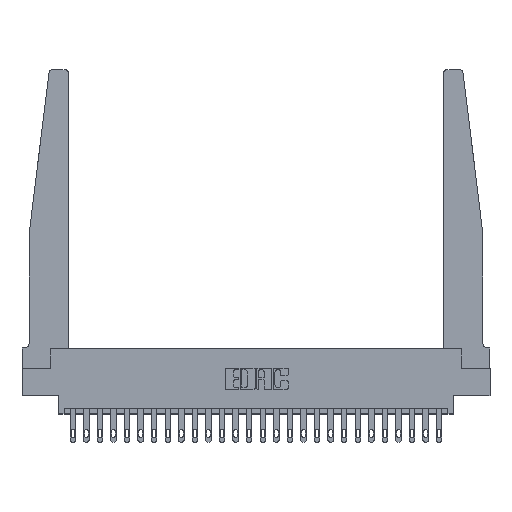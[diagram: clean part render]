
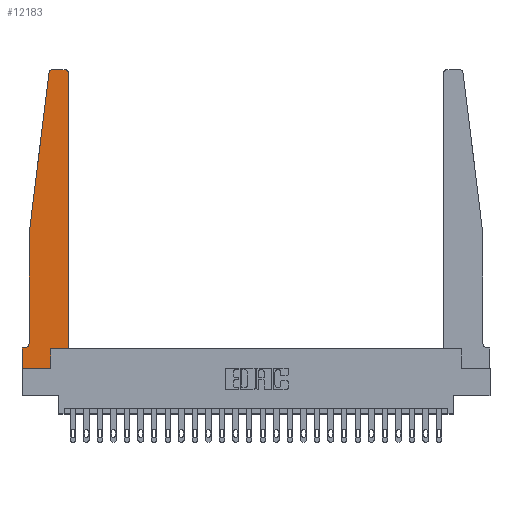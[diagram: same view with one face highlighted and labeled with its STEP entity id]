
A CAD part, top view. The second image highlights one B-rep face of the part: STEP entity #12183.
In plain terms, the highlighted planar face has unit normal (0, 0, 1).
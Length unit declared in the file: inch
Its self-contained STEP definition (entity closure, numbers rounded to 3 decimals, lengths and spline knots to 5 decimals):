
#21 = VECTOR ( 'NONE', #12403, 39.37008 ) ;
#316 = DIRECTION ( 'NONE',  ( 0., -1., 0. ) ) ;
#519 = VERTEX_POINT ( 'NONE', #16243 ) ;
#583 = VECTOR ( 'NONE', #2720, 39.37008 ) ;
#841 = ORIENTED_EDGE ( 'NONE', *, *, #5071, .T. ) ;
#879 = LINE ( 'NONE', #22635, #21383 ) ;
#904 = CARTESIAN_POINT ( 'NONE',  ( 0.2605, 0.18, 0.37 ) ) ;
#988 = CARTESIAN_POINT ( 'NONE',  ( 0.065, 1.25, 0.37 ) ) ;
#1230 = CARTESIAN_POINT ( 'NONE',  ( 0.425, 0.18, 0.37 ) ) ;
#1241 = ORIENTED_EDGE ( 'NONE', *, *, #4500, .T. ) ;
#1388 = CIRCLE ( 'NONE', #5923, 0.05 ) ;
#1727 = CARTESIAN_POINT ( 'NONE',  ( 0.27653, 2.72, 0.37 ) ) ;
#1816 = LINE ( 'NONE', #7747, #4727 ) ;
#1853 = EDGE_CURVE ( 'NONE', #3361, #12237, #2356, .T. ) ;
#2356 = LINE ( 'NONE', #21667, #24322 ) ;
#2442 = CARTESIAN_POINT ( 'NONE',  ( 0.065, 1.25, 0.37 ) ) ;
#2459 = LINE ( 'NONE', #904, #8389 ) ;
#2460 = FACE_OUTER_BOUND ( 'NONE', #20268, .T. ) ;
#2645 = AXIS2_PLACEMENT_3D ( 'NONE', #1727, #7530, #21415 ) ;
#2720 = DIRECTION ( 'NONE',  ( 0., 1., 0. ) ) ;
#3138 = VERTEX_POINT ( 'NONE', #988 ) ;
#3288 = ORIENTED_EDGE ( 'NONE', *, *, #16578, .T. ) ;
#3361 = VERTEX_POINT ( 'NONE', #10367 ) ;
#3386 = DIRECTION ( 'NONE',  ( 0., 0., 1. ) ) ;
#3584 = EDGE_CURVE ( 'NONE', #12237, #519, #18254, .T. ) ;
#3798 = CARTESIAN_POINT ( 'NONE',  ( 0.065, 0.1875, 0.37 ) ) ;
#3959 = VECTOR ( 'NONE', #316, 39.37008 ) ;
#4500 = EDGE_CURVE ( 'NONE', #24695, #19992, #1388, .T. ) ;
#4727 = VECTOR ( 'NONE', #9683, 39.37008 ) ;
#4728 = LINE ( 'NONE', #1230, #13817 ) ;
#5071 = EDGE_CURVE ( 'NONE', #15024, #10691, #21679, .T. ) ;
#5421 = CARTESIAN_POINT ( 'NONE',  ( 0.2605, 0., 0.37 ) ) ;
#5449 = EDGE_CURVE ( 'NONE', #9750, #23066, #2459, .T. ) ;
#5635 = DIRECTION ( 'NONE',  ( 0., 0., -1. ) ) ;
#5793 = CIRCLE ( 'NONE', #16869, 0.03 ) ;
#5923 = AXIS2_PLACEMENT_3D ( 'NONE', #23272, #5635, #13356 ) ;
#6958 = DIRECTION ( 'NONE',  ( 0., 1., 0. ) ) ;
#7075 = ORIENTED_EDGE ( 'NONE', *, *, #1853, .T. ) ;
#7202 = EDGE_CURVE ( 'NONE', #10691, #9750, #879, .T. ) ;
#7530 = DIRECTION ( 'NONE',  ( 0., 0., 1. ) ) ;
#7678 = LINE ( 'NONE', #3798, #21 ) ;
#7747 = CARTESIAN_POINT ( 'NONE',  ( 0.065, 1.25, 0.37 ) ) ;
#7836 = VERTEX_POINT ( 'NONE', #13845 ) ;
#8345 = ORIENTED_EDGE ( 'NONE', *, *, #9409, .T. ) ;
#8379 = DIRECTION ( 'NONE',  ( 0., 0., 1. ) ) ;
#8389 = VECTOR ( 'NONE', #6958, 39.37008 ) ;
#8492 = CARTESIAN_POINT ( 'NONE',  ( 0.425, 2.72, 0.37 ) ) ;
#8969 = EDGE_CURVE ( 'NONE', #19992, #15024, #7678, .T. ) ;
#9033 = CARTESIAN_POINT ( 'NONE',  ( 0.2605, 0.18, 0.37 ) ) ;
#9105 = DIRECTION ( 'NONE',  ( 1., 0., 0. ) ) ;
#9409 = EDGE_CURVE ( 'NONE', #10160, #3361, #5793, .T. ) ;
#9436 = ORIENTED_EDGE ( 'NONE', *, *, #3584, .T. ) ;
#9683 = DIRECTION ( 'NONE',  ( 0., -1., 0. ) ) ;
#9750 = VERTEX_POINT ( 'NONE', #5421 ) ;
#9835 = CARTESIAN_POINT ( 'NONE',  ( 0.065, 0.2375, 0.37 ) ) ;
#10160 = VERTEX_POINT ( 'NONE', #8492 ) ;
#10367 = CARTESIAN_POINT ( 'NONE',  ( 0.395, 2.75, 0.37 ) ) ;
#10691 = VERTEX_POINT ( 'NONE', #19606 ) ;
#11228 = DIRECTION ( 'NONE',  ( 1., 0., 0. ) ) ;
#12183 = ADVANCED_FACE ( 'NONE', ( #2460 ), #22145, .T. ) ;
#12237 = VERTEX_POINT ( 'NONE', #18529 ) ;
#12403 = DIRECTION ( 'NONE',  ( -1., 0., 0. ) ) ;
#12491 = LINE ( 'NONE', #16235, #583 ) ;
#12718 = DIRECTION ( 'NONE',  ( 1., 0., 0. ) ) ;
#13166 = CARTESIAN_POINT ( 'NONE',  ( 0.395, 2.72, 0.37 ) ) ;
#13356 = DIRECTION ( 'NONE',  ( -1., 0., 0. ) ) ;
#13361 = EDGE_CURVE ( 'NONE', #7836, #10160, #12491, .T. ) ;
#13817 = VECTOR ( 'NONE', #9105, 39.37008 ) ;
#13845 = CARTESIAN_POINT ( 'NONE',  ( 0.425, 0.18, 0.37 ) ) ;
#13904 = LINE ( 'NONE', #2442, #16758 ) ;
#15024 = VERTEX_POINT ( 'NONE', #16491 ) ;
#16235 = CARTESIAN_POINT ( 'NONE',  ( 0.425, 0.18, 0.37 ) ) ;
#16243 = CARTESIAN_POINT ( 'NONE',  ( 0.24675, 2.72367, 0.37 ) ) ;
#16491 = CARTESIAN_POINT ( 'NONE',  ( 0., 0.1875, 0.37 ) ) ;
#16578 = EDGE_CURVE ( 'NONE', #3138, #24695, #1816, .T. ) ;
#16758 = VECTOR ( 'NONE', #23944, 39.37008 ) ;
#16840 = CARTESIAN_POINT ( 'NONE',  ( 0.015, 0.1875, 0.37 ) ) ;
#16869 = AXIS2_PLACEMENT_3D ( 'NONE', #13166, #3386, #11228 ) ;
#17090 = DIRECTION ( 'NONE',  ( 1., 0., 0. ) ) ;
#17307 = EDGE_CURVE ( 'NONE', #23066, #7836, #4728, .T. ) ;
#17940 = CARTESIAN_POINT ( 'NONE',  ( 0., 0., 0.37 ) ) ;
#18254 = CIRCLE ( 'NONE', #2645, 0.03 ) ;
#18529 = CARTESIAN_POINT ( 'NONE',  ( 0.27653, 2.75, 0.37 ) ) ;
#19606 = CARTESIAN_POINT ( 'NONE',  ( 0., 0., 0.37 ) ) ;
#19772 = EDGE_CURVE ( 'NONE', #519, #3138, #13904, .T. ) ;
#19992 = VERTEX_POINT ( 'NONE', #16840 ) ;
#20241 = AXIS2_PLACEMENT_3D ( 'NONE', #22026, #8379, #17090 ) ;
#20268 = EDGE_LOOP ( 'NONE', ( #7075, #9436, #23771, #3288, #1241, #21312, #841, #22679, #25283, #23312, #25217, #8345 ) ) ;
#21312 = ORIENTED_EDGE ( 'NONE', *, *, #8969, .T. ) ;
#21383 = VECTOR ( 'NONE', #12718, 39.37008 ) ;
#21415 = DIRECTION ( 'NONE',  ( 1., 0., 0. ) ) ;
#21539 = DIRECTION ( 'NONE',  ( -1., 0., 0. ) ) ;
#21667 = CARTESIAN_POINT ( 'NONE',  ( 0.25, 2.75, 0.37 ) ) ;
#21679 = LINE ( 'NONE', #17940, #3959 ) ;
#22026 = CARTESIAN_POINT ( 'NONE',  ( 0., 0.1875, 0.37 ) ) ;
#22145 = PLANE ( 'NONE',  #20241 ) ;
#22635 = CARTESIAN_POINT ( 'NONE',  ( 0., 0., 0.37 ) ) ;
#22679 = ORIENTED_EDGE ( 'NONE', *, *, #7202, .T. ) ;
#23066 = VERTEX_POINT ( 'NONE', #9033 ) ;
#23272 = CARTESIAN_POINT ( 'NONE',  ( 0.015, 0.2375, 0.37 ) ) ;
#23312 = ORIENTED_EDGE ( 'NONE', *, *, #17307, .T. ) ;
#23771 = ORIENTED_EDGE ( 'NONE', *, *, #19772, .T. ) ;
#23944 = DIRECTION ( 'NONE',  ( -0.122, -0.992, 0. ) ) ;
#24322 = VECTOR ( 'NONE', #21539, 39.37008 ) ;
#24695 = VERTEX_POINT ( 'NONE', #9835 ) ;
#25217 = ORIENTED_EDGE ( 'NONE', *, *, #13361, .T. ) ;
#25283 = ORIENTED_EDGE ( 'NONE', *, *, #5449, .T. ) ;
